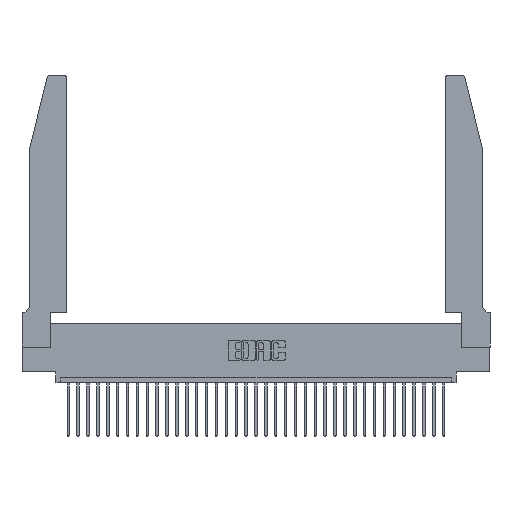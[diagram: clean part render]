
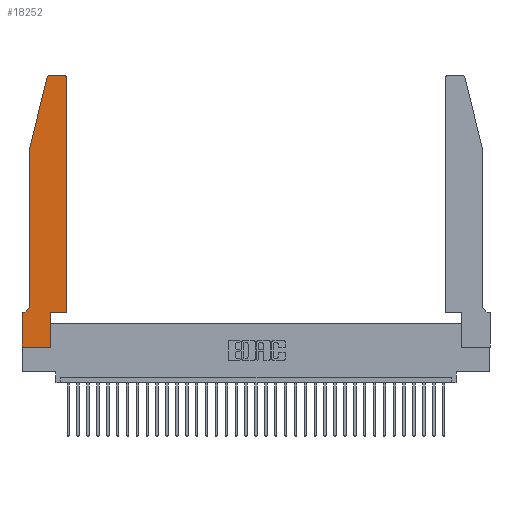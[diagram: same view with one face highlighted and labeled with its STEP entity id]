
A CAD part, top view. The second image highlights one B-rep face of the part: STEP entity #18252.
In plain terms, the highlighted planar face has unit normal (0, 0, 1).
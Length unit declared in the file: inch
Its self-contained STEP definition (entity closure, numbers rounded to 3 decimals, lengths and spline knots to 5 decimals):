
#17 = ORIENTED_EDGE ( 'NONE', *, *, #3024, .T. ) ;
#396 = ORIENTED_EDGE ( 'NONE', *, *, #25356, .T. ) ;
#630 = VECTOR ( 'NONE', #15195, 39.37008 ) ;
#671 = DIRECTION ( 'NONE',  ( 1., 0., 0. ) ) ;
#1074 = CARTESIAN_POINT ( 'NONE',  ( 0.0055, 0.35, 0.37 ) ) ;
#1881 = CARTESIAN_POINT ( 'NONE',  ( 0.0755, 2., 0.37 ) ) ;
#2190 = ORIENTED_EDGE ( 'NONE', *, *, #12300, .T. ) ;
#2340 = DIRECTION ( 'NONE',  ( -1., 0., 0. ) ) ;
#2436 = VECTOR ( 'NONE', #31226, 39.37008 ) ;
#2563 = EDGE_CURVE ( 'NONE', #6049, #27670, #10345, .T. ) ;
#3024 = EDGE_CURVE ( 'NONE', #6676, #14456, #21631, .T. ) ;
#3442 = CARTESIAN_POINT ( 'NONE',  ( 0.2865, 0., 0.37 ) ) ;
#3605 = DIRECTION ( 'NONE',  ( 0., 0., 1. ) ) ;
#3774 = EDGE_CURVE ( 'NONE', #4754, #12486, #16952, .T. ) ;
#4754 = VERTEX_POINT ( 'NONE', #15831 ) ;
#4877 = VECTOR ( 'NONE', #33001, 39.37008 ) ;
#4989 = CARTESIAN_POINT ( 'NONE',  ( 0.0755, 2., 0.37 ) ) ;
#5037 = CIRCLE ( 'NONE', #11283, 0.03 ) ;
#5117 = DIRECTION ( 'NONE',  ( 0., 0., -1. ) ) ;
#5815 = EDGE_CURVE ( 'NONE', #9934, #33624, #23964, .T. ) ;
#5988 = CIRCLE ( 'NONE', #18676, 0.03 ) ;
#6008 = CARTESIAN_POINT ( 'NONE',  ( 0.4505, 2.72, 0.37 ) ) ;
#6049 = VERTEX_POINT ( 'NONE', #23998 ) ;
#6676 = VERTEX_POINT ( 'NONE', #21882 ) ;
#6704 = DIRECTION ( 'NONE',  ( 1., 0., 0. ) ) ;
#7213 = EDGE_LOOP ( 'NONE', ( #17, #14691, #29063, #19615, #31222, #2190, #30364, #396, #28765, #29780, #15776, #8011 ) ) ;
#7252 = EDGE_CURVE ( 'NONE', #8706, #32508, #23913, .T. ) ;
#7370 = VERTEX_POINT ( 'NONE', #3442 ) ;
#7703 = CARTESIAN_POINT ( 'NONE',  ( 0.284, 2.75, 0.37 ) ) ;
#7870 = DIRECTION ( 'NONE',  ( 0., -1., 0. ) ) ;
#8011 = ORIENTED_EDGE ( 'NONE', *, *, #25584, .T. ) ;
#8706 = VERTEX_POINT ( 'NONE', #12781 ) ;
#8764 = CARTESIAN_POINT ( 'NONE',  ( 0.4505, 0.35, 0.37 ) ) ;
#9237 = DIRECTION ( 'NONE',  ( 0., 0., 1. ) ) ;
#9934 = VERTEX_POINT ( 'NONE', #16034 ) ;
#10121 = LINE ( 'NONE', #25288, #23166 ) ;
#10345 = LINE ( 'NONE', #12464, #17902 ) ;
#10525 = VECTOR ( 'NONE', #33822, 39.37008 ) ;
#11283 = AXIS2_PLACEMENT_3D ( 'NONE', #14533, #9237, #671 ) ;
#11735 = EDGE_CURVE ( 'NONE', #7370, #6049, #22536, .T. ) ;
#11835 = CARTESIAN_POINT ( 'NONE',  ( 0.284, 2.72, 0.37 ) ) ;
#12300 = EDGE_CURVE ( 'NONE', #12486, #8706, #14986, .T. ) ;
#12464 = CARTESIAN_POINT ( 'NONE',  ( 0.4505, 0.35, 0.37 ) ) ;
#12486 = VERTEX_POINT ( 'NONE', #1074 ) ;
#12781 = CARTESIAN_POINT ( 'NONE',  ( 0., 0.35, 0.37 ) ) ;
#12884 = CARTESIAN_POINT ( 'NONE',  ( 0.0055, 0.42, 0.37 ) ) ;
#13447 = EDGE_CURVE ( 'NONE', #14456, #9934, #5988, .T. ) ;
#13861 = CARTESIAN_POINT ( 'NONE',  ( 0.4505, 0.35, 0.37 ) ) ;
#13996 = DIRECTION ( 'NONE',  ( 0., -1., 0. ) ) ;
#14456 = VERTEX_POINT ( 'NONE', #7703 ) ;
#14522 = VECTOR ( 'NONE', #29420, 39.37008 ) ;
#14533 = CARTESIAN_POINT ( 'NONE',  ( 0.4205, 2.72, 0.37 ) ) ;
#14691 = ORIENTED_EDGE ( 'NONE', *, *, #13447, .T. ) ;
#14986 = LINE ( 'NONE', #28241, #4877 ) ;
#15085 = VECTOR ( 'NONE', #7870, 39.37008 ) ;
#15195 = DIRECTION ( 'NONE',  ( 0., 1., 0. ) ) ;
#15776 = ORIENTED_EDGE ( 'NONE', *, *, #29695, .T. ) ;
#15831 = CARTESIAN_POINT ( 'NONE',  ( 0.0755, 0.42, 0.37 ) ) ;
#16034 = CARTESIAN_POINT ( 'NONE',  ( 0.25487, 2.72718, 0.37 ) ) ;
#16952 = CIRCLE ( 'NONE', #28512, 0.07 ) ;
#16993 = LINE ( 'NONE', #8764, #630 ) ;
#17207 = CARTESIAN_POINT ( 'NONE',  ( 0.0755, 2., 0.37 ) ) ;
#17902 = VECTOR ( 'NONE', #6704, 39.37008 ) ;
#18252 = ADVANCED_FACE ( 'NONE', ( #25194 ), #21699, .T. ) ;
#18676 = AXIS2_PLACEMENT_3D ( 'NONE', #11835, #33242, #27444 ) ;
#19615 = ORIENTED_EDGE ( 'NONE', *, *, #22537, .T. ) ;
#21631 = LINE ( 'NONE', #31082, #14522 ) ;
#21699 = PLANE ( 'NONE',  #31362 ) ;
#21882 = CARTESIAN_POINT ( 'NONE',  ( 0.4205, 2.75, 0.37 ) ) ;
#22536 = LINE ( 'NONE', #24974, #2436 ) ;
#22537 = EDGE_CURVE ( 'NONE', #33624, #4754, #31206, .T. ) ;
#22703 = DIRECTION ( 'NONE',  ( 1., 0., 0. ) ) ;
#23166 = VECTOR ( 'NONE', #22703, 39.37008 ) ;
#23409 = CARTESIAN_POINT ( 'NONE',  ( 0., 0., 0.37 ) ) ;
#23913 = LINE ( 'NONE', #26746, #15085 ) ;
#23964 = LINE ( 'NONE', #1881, #10525 ) ;
#23998 = CARTESIAN_POINT ( 'NONE',  ( 0.2865, 0.35, 0.37 ) ) ;
#24943 = VECTOR ( 'NONE', #13996, 39.37008 ) ;
#24974 = CARTESIAN_POINT ( 'NONE',  ( 0.2865, 0.35, 0.37 ) ) ;
#25194 = FACE_OUTER_BOUND ( 'NONE', #7213, .T. ) ;
#25231 = DIRECTION ( 'NONE',  ( 1., 0., 0. ) ) ;
#25288 = CARTESIAN_POINT ( 'NONE',  ( 0., 0., 0.37 ) ) ;
#25356 = EDGE_CURVE ( 'NONE', #32508, #7370, #10121, .T. ) ;
#25584 = EDGE_CURVE ( 'NONE', #31272, #6676, #5037, .T. ) ;
#26746 = CARTESIAN_POINT ( 'NONE',  ( 0., 0., 0.37 ) ) ;
#27444 = DIRECTION ( 'NONE',  ( 1., 0., 0. ) ) ;
#27670 = VERTEX_POINT ( 'NONE', #13861 ) ;
#28241 = CARTESIAN_POINT ( 'NONE',  ( 0.0755, 0.35, 0.37 ) ) ;
#28512 = AXIS2_PLACEMENT_3D ( 'NONE', #12884, #5117, #2340 ) ;
#28765 = ORIENTED_EDGE ( 'NONE', *, *, #11735, .T. ) ;
#29063 = ORIENTED_EDGE ( 'NONE', *, *, #5815, .T. ) ;
#29420 = DIRECTION ( 'NONE',  ( -1., 0., 0. ) ) ;
#29695 = EDGE_CURVE ( 'NONE', #27670, #31272, #16993, .T. ) ;
#29780 = ORIENTED_EDGE ( 'NONE', *, *, #2563, .T. ) ;
#29997 = CARTESIAN_POINT ( 'NONE',  ( 0., 0.35, 0.37 ) ) ;
#30364 = ORIENTED_EDGE ( 'NONE', *, *, #7252, .T. ) ;
#31082 = CARTESIAN_POINT ( 'NONE',  ( 0.2605, 2.75, 0.37 ) ) ;
#31206 = LINE ( 'NONE', #4989, #24943 ) ;
#31222 = ORIENTED_EDGE ( 'NONE', *, *, #3774, .T. ) ;
#31226 = DIRECTION ( 'NONE',  ( 0., 1., 0. ) ) ;
#31272 = VERTEX_POINT ( 'NONE', #6008 ) ;
#31362 = AXIS2_PLACEMENT_3D ( 'NONE', #29997, #3605, #25231 ) ;
#32508 = VERTEX_POINT ( 'NONE', #23409 ) ;
#33001 = DIRECTION ( 'NONE',  ( -1., 0., 0. ) ) ;
#33242 = DIRECTION ( 'NONE',  ( 0., 0., 1. ) ) ;
#33624 = VERTEX_POINT ( 'NONE', #17207 ) ;
#33822 = DIRECTION ( 'NONE',  ( -0.239, -0.971, 0. ) ) ;
